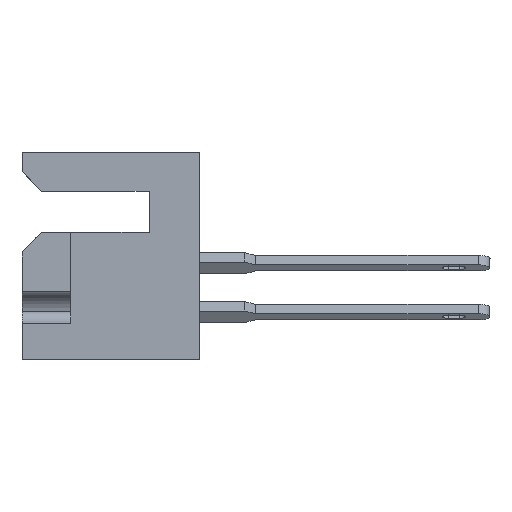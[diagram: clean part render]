
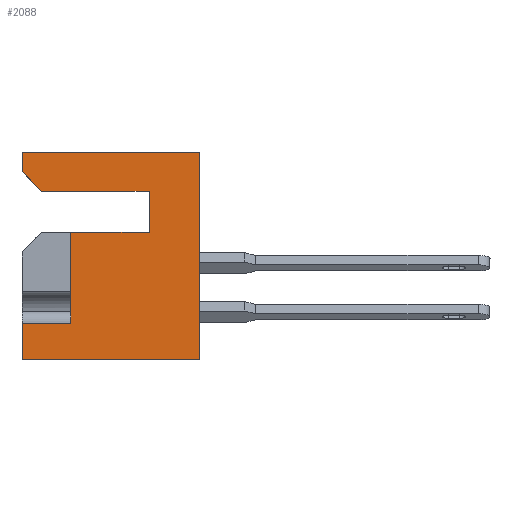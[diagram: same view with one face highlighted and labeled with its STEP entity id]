
A CAD part, left-side view. The second image highlights one B-rep face of the part: STEP entity #2088.
In plain terms, the highlighted planar face has unit normal (-1, 0, 0).
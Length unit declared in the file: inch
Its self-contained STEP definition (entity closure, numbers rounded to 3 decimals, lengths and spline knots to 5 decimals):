
#237 = DIRECTION ( 'NONE',  ( 0., -0.707, -0.707 ) ) ;
#270 = VERTEX_POINT ( 'NONE', #16093 ) ;
#396 = VERTEX_POINT ( 'NONE', #2221 ) ;
#525 = AXIS2_PLACEMENT_3D ( 'NONE', #9018, #5292, #2725 ) ;
#536 = CARTESIAN_POINT ( 'NONE',  ( 0., 0.403, -0.1 ) ) ;
#648 = VECTOR ( 'NONE', #11494, 39.37008 ) ;
#699 = LINE ( 'NONE', #13341, #7857 ) ;
#977 = EDGE_LOOP ( 'NONE', ( #12350, #4551, #1184, #12325, #11801, #8926, #4876, #9386, #7537, #2249, #11133 ) ) ;
#1184 = ORIENTED_EDGE ( 'NONE', *, *, #3243, .T. ) ;
#1543 = CARTESIAN_POINT ( 'NONE',  ( 0., 0.453, 0. ) ) ;
#1785 = LINE ( 'NONE', #5989, #3962 ) ;
#1949 = VECTOR ( 'NONE', #9310, 39.37008 ) ;
#2088 = ADVANCED_FACE ( 'NONE', ( #12597 ), #12990, .F. ) ;
#2138 = CARTESIAN_POINT ( 'NONE',  ( 0., 0., 0. ) ) ;
#2221 = CARTESIAN_POINT ( 'NONE',  ( 0., 0.453, -0.05 ) ) ;
#2249 = ORIENTED_EDGE ( 'NONE', *, *, #3790, .T. ) ;
#2283 = LINE ( 'NONE', #16215, #8226 ) ;
#2532 = CARTESIAN_POINT ( 'NONE',  ( 0., 0.328, -0.437 ) ) ;
#2676 = VERTEX_POINT ( 'NONE', #3501 ) ;
#2696 = VECTOR ( 'NONE', #2738, 39.37008 ) ;
#2725 = DIRECTION ( 'NONE',  ( 0., 0., -1. ) ) ;
#2738 = DIRECTION ( 'NONE',  ( 0., 1., 0. ) ) ;
#2786 = CARTESIAN_POINT ( 'NONE',  ( 0., 0.128, -0.205 ) ) ;
#2957 = LINE ( 'NONE', #14580, #3767 ) ;
#3243 = EDGE_CURVE ( 'NONE', #8161, #4678, #11160, .T. ) ;
#3254 = DIRECTION ( 'NONE',  ( 0., 0., 1. ) ) ;
#3501 = CARTESIAN_POINT ( 'NONE',  ( 0., 0.328, -0.205 ) ) ;
#3521 = LINE ( 'NONE', #15491, #1949 ) ;
#3639 = EDGE_CURVE ( 'NONE', #13522, #7335, #2957, .T. ) ;
#3767 = VECTOR ( 'NONE', #15826, 39.37008 ) ;
#3790 = EDGE_CURVE ( 'NONE', #11193, #2676, #10937, .T. ) ;
#3962 = VECTOR ( 'NONE', #14923, 39.37008 ) ;
#4160 = VECTOR ( 'NONE', #15180, 39.37008 ) ;
#4394 = CARTESIAN_POINT ( 'NONE',  ( 0., 0., -0.531 ) ) ;
#4551 = ORIENTED_EDGE ( 'NONE', *, *, #13556, .F. ) ;
#4678 = VERTEX_POINT ( 'NONE', #4394 ) ;
#4870 = VECTOR ( 'NONE', #3254, 39.37008 ) ;
#4876 = ORIENTED_EDGE ( 'NONE', *, *, #10505, .T. ) ;
#5292 = DIRECTION ( 'NONE',  ( 1., 0., 0. ) ) ;
#5974 = CARTESIAN_POINT ( 'NONE',  ( 0., 0.328, -0.437 ) ) ;
#5989 = CARTESIAN_POINT ( 'NONE',  ( 0., 0.453, 0. ) ) ;
#6368 = VECTOR ( 'NONE', #11191, 39.37008 ) ;
#6875 = EDGE_CURVE ( 'NONE', #10131, #2676, #699, .T. ) ;
#7049 = VECTOR ( 'NONE', #237, 39.37008 ) ;
#7335 = VERTEX_POINT ( 'NONE', #536 ) ;
#7480 = CARTESIAN_POINT ( 'NONE',  ( 0., 0.453, -0.531 ) ) ;
#7537 = ORIENTED_EDGE ( 'NONE', *, *, #8828, .F. ) ;
#7671 = CARTESIAN_POINT ( 'NONE',  ( 0., 0.453, 0. ) ) ;
#7857 = VECTOR ( 'NONE', #15964, 39.37008 ) ;
#8161 = VERTEX_POINT ( 'NONE', #7480 ) ;
#8226 = VECTOR ( 'NONE', #9497, 39.37008 ) ;
#8828 = EDGE_CURVE ( 'NONE', #11193, #13522, #3521, .T. ) ;
#8926 = ORIENTED_EDGE ( 'NONE', *, *, #11107, .F. ) ;
#9018 = CARTESIAN_POINT ( 'NONE',  ( 0., 0.453, 0. ) ) ;
#9310 = DIRECTION ( 'NONE',  ( 0., 0., 1. ) ) ;
#9386 = ORIENTED_EDGE ( 'NONE', *, *, #3639, .F. ) ;
#9497 = DIRECTION ( 'NONE',  ( 0., -1., 0. ) ) ;
#10065 = CARTESIAN_POINT ( 'NONE',  ( 0., 0.453, -0.531 ) ) ;
#10118 = CARTESIAN_POINT ( 'NONE',  ( 0., 0.128, -0.205 ) ) ;
#10131 = VERTEX_POINT ( 'NONE', #5974 ) ;
#10146 = EDGE_CURVE ( 'NONE', #4678, #12858, #15862, .T. ) ;
#10406 = LINE ( 'NONE', #7671, #648 ) ;
#10431 = EDGE_CURVE ( 'NONE', #10131, #270, #14075, .T. ) ;
#10505 = EDGE_CURVE ( 'NONE', #396, #7335, #14442, .T. ) ;
#10937 = LINE ( 'NONE', #10118, #4160 ) ;
#11030 = CARTESIAN_POINT ( 'NONE',  ( 0., 0., 0. ) ) ;
#11107 = EDGE_CURVE ( 'NONE', #396, #16140, #10406, .T. ) ;
#11133 = ORIENTED_EDGE ( 'NONE', *, *, #6875, .F. ) ;
#11160 = LINE ( 'NONE', #10065, #6368 ) ;
#11191 = DIRECTION ( 'NONE',  ( 0., -1., 0. ) ) ;
#11193 = VERTEX_POINT ( 'NONE', #2786 ) ;
#11494 = DIRECTION ( 'NONE',  ( 0., 0., 1. ) ) ;
#11801 = ORIENTED_EDGE ( 'NONE', *, *, #14558, .F. ) ;
#12325 = ORIENTED_EDGE ( 'NONE', *, *, #10146, .T. ) ;
#12350 = ORIENTED_EDGE ( 'NONE', *, *, #10431, .T. ) ;
#12597 = FACE_OUTER_BOUND ( 'NONE', #977, .T. ) ;
#12784 = CARTESIAN_POINT ( 'NONE',  ( 0., 0.403, -0.1 ) ) ;
#12858 = VERTEX_POINT ( 'NONE', #11030 ) ;
#12990 = PLANE ( 'NONE',  #525 ) ;
#13341 = CARTESIAN_POINT ( 'NONE',  ( 0., 0.328, -0.205 ) ) ;
#13522 = VERTEX_POINT ( 'NONE', #14880 ) ;
#13556 = EDGE_CURVE ( 'NONE', #8161, #270, #1785, .T. ) ;
#14075 = LINE ( 'NONE', #2532, #2696 ) ;
#14442 = LINE ( 'NONE', #12784, #7049 ) ;
#14558 = EDGE_CURVE ( 'NONE', #16140, #12858, #2283, .T. ) ;
#14580 = CARTESIAN_POINT ( 'NONE',  ( 0., 0.128, -0.1 ) ) ;
#14880 = CARTESIAN_POINT ( 'NONE',  ( 0., 0.128, -0.1 ) ) ;
#14923 = DIRECTION ( 'NONE',  ( 0., 0., 1. ) ) ;
#15180 = DIRECTION ( 'NONE',  ( 0., 1., 0. ) ) ;
#15491 = CARTESIAN_POINT ( 'NONE',  ( 0., 0.128, -0.1 ) ) ;
#15826 = DIRECTION ( 'NONE',  ( 0., 1., 0. ) ) ;
#15862 = LINE ( 'NONE', #2138, #4870 ) ;
#15964 = DIRECTION ( 'NONE',  ( 0., 0., 1. ) ) ;
#16093 = CARTESIAN_POINT ( 'NONE',  ( 0., 0.453, -0.437 ) ) ;
#16140 = VERTEX_POINT ( 'NONE', #1543 ) ;
#16215 = CARTESIAN_POINT ( 'NONE',  ( 0., 0.453, 0. ) ) ;
